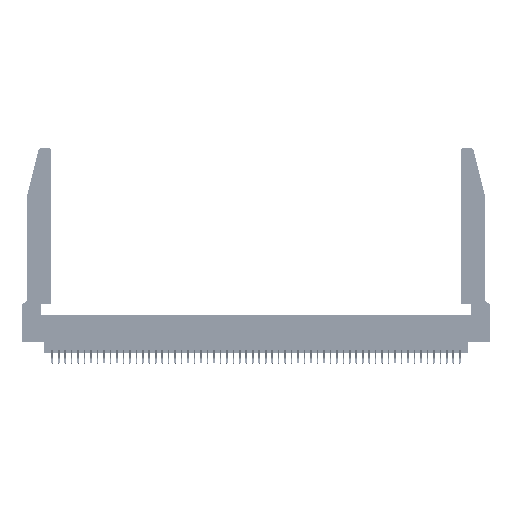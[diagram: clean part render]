
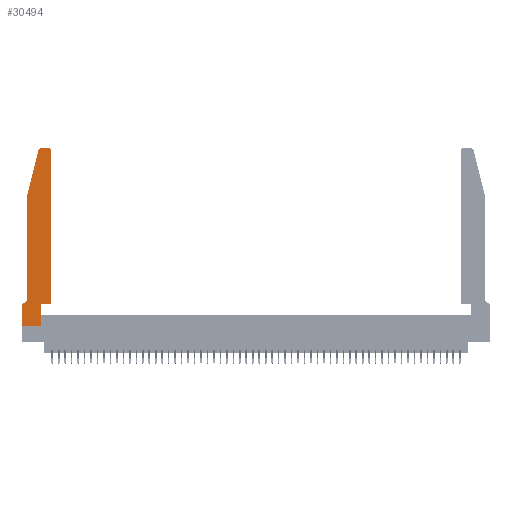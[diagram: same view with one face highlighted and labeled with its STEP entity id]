
A CAD part, top view. The second image highlights one B-rep face of the part: STEP entity #30494.
In plain terms, the highlighted planar face has unit normal (0, 0, 1).
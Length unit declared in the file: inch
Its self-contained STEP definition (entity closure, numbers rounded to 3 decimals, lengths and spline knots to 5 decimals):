
#531 = EDGE_CURVE ( 'NONE', #18446, #40915, #42597, .T. ) ;
#561 = ORIENTED_EDGE ( 'NONE', *, *, #23135, .T. ) ;
#687 = ORIENTED_EDGE ( 'NONE', *, *, #11111, .T. ) ;
#2513 = ORIENTED_EDGE ( 'NONE', *, *, #46568, .T. ) ;
#2864 = LINE ( 'NONE', #10462, #12907 ) ;
#4147 = CIRCLE ( 'NONE', #18333, 0.07 ) ;
#4244 = VECTOR ( 'NONE', #49688, 39.37008 ) ;
#4276 = DIRECTION ( 'NONE',  ( 0., 1., 0. ) ) ;
#4467 = CARTESIAN_POINT ( 'NONE',  ( 0.4205, 2.72, 0.37 ) ) ;
#5077 = CARTESIAN_POINT ( 'NONE',  ( 0.0755, 0.35, 0.37 ) ) ;
#5909 = VECTOR ( 'NONE', #18284, 39.37008 ) ;
#6375 = ORIENTED_EDGE ( 'NONE', *, *, #531, .T. ) ;
#6644 = AXIS2_PLACEMENT_3D ( 'NONE', #11214, #19170, #7177 ) ;
#6921 = DIRECTION ( 'NONE',  ( 1., 0., 0. ) ) ;
#7177 = DIRECTION ( 'NONE',  ( 1., 0., 0. ) ) ;
#7251 = ORIENTED_EDGE ( 'NONE', *, *, #20169, .T. ) ;
#7754 = CARTESIAN_POINT ( 'NONE',  ( 0.4505, 0.35, 0.37 ) ) ;
#7793 = EDGE_CURVE ( 'NONE', #28398, #52288, #38190, .T. ) ;
#8752 = CARTESIAN_POINT ( 'NONE',  ( 0., 0.35, 0.37 ) ) ;
#10229 = VERTEX_POINT ( 'NONE', #35747 ) ;
#10462 = CARTESIAN_POINT ( 'NONE',  ( 0., 0., 0.37 ) ) ;
#11111 = EDGE_CURVE ( 'NONE', #30848, #43019, #2864, .T. ) ;
#11214 = CARTESIAN_POINT ( 'NONE',  ( 0., 0.35, 0.37 ) ) ;
#12907 = VECTOR ( 'NONE', #23030, 39.37008 ) ;
#13020 = DIRECTION ( 'NONE',  ( -1., 0., 0. ) ) ;
#13340 = ORIENTED_EDGE ( 'NONE', *, *, #48735, .T. ) ;
#15078 = VECTOR ( 'NONE', #4276, 39.37008 ) ;
#15363 = CARTESIAN_POINT ( 'NONE',  ( 0.0755, 2., 0.37 ) ) ;
#16122 = CARTESIAN_POINT ( 'NONE',  ( 0.0755, 2., 0.37 ) ) ;
#16794 = EDGE_CURVE ( 'NONE', #52288, #40563, #49364, .T. ) ;
#16903 = EDGE_CURVE ( 'NONE', #34697, #10229, #19026, .T. ) ;
#18088 = LINE ( 'NONE', #5077, #35847 ) ;
#18284 = DIRECTION ( 'NONE',  ( 0., 1., 0. ) ) ;
#18333 = AXIS2_PLACEMENT_3D ( 'NONE', #35496, #46964, #51045 ) ;
#18446 = VERTEX_POINT ( 'NONE', #7754 ) ;
#18973 = CARTESIAN_POINT ( 'NONE',  ( 0.4505, 0.35, 0.37 ) ) ;
#19026 = LINE ( 'NONE', #41815, #30391 ) ;
#19170 = DIRECTION ( 'NONE',  ( 0., 0., 1. ) ) ;
#20121 = ORIENTED_EDGE ( 'NONE', *, *, #16794, .T. ) ;
#20169 = EDGE_CURVE ( 'NONE', #41918, #18446, #46542, .T. ) ;
#20224 = DIRECTION ( 'NONE',  ( -0.239, -0.971, 0. ) ) ;
#22528 = CARTESIAN_POINT ( 'NONE',  ( 0.0055, 0.35, 0.37 ) ) ;
#22739 = CARTESIAN_POINT ( 'NONE',  ( 0.2865, 0.35, 0.37 ) ) ;
#22975 = VECTOR ( 'NONE', #20224, 39.37008 ) ;
#23030 = DIRECTION ( 'NONE',  ( 1., 0., 0. ) ) ;
#23135 = EDGE_CURVE ( 'NONE', #46210, #30848, #42848, .T. ) ;
#23597 = PLANE ( 'NONE',  #6644 ) ;
#24251 = EDGE_CURVE ( 'NONE', #40563, #48288, #4147, .T. ) ;
#24945 = DIRECTION ( 'NONE',  ( 0., 0., 1. ) ) ;
#25653 = VECTOR ( 'NONE', #6921, 39.37008 ) ;
#26366 = AXIS2_PLACEMENT_3D ( 'NONE', #4467, #24945, #44942 ) ;
#26538 = DIRECTION ( 'NONE',  ( 0., -1., 0. ) ) ;
#27041 = CARTESIAN_POINT ( 'NONE',  ( 0.4505, 0.35, 0.37 ) ) ;
#27242 = ORIENTED_EDGE ( 'NONE', *, *, #51098, .T. ) ;
#28184 = EDGE_LOOP ( 'NONE', ( #50479, #2513, #41873, #20121, #33428, #27242, #561, #687, #13340, #7251, #6375, #51823 ) ) ;
#28398 = VERTEX_POINT ( 'NONE', #32281 ) ;
#28802 = CARTESIAN_POINT ( 'NONE',  ( 0., 0., 0.37 ) ) ;
#30045 = CARTESIAN_POINT ( 'NONE',  ( 0.0755, 0.42, 0.37 ) ) ;
#30391 = VECTOR ( 'NONE', #46049, 39.37008 ) ;
#30486 = CARTESIAN_POINT ( 'NONE',  ( 0.284, 2.72, 0.37 ) ) ;
#30494 = ADVANCED_FACE ( 'NONE', ( #31846 ), #23597, .T. ) ;
#30787 = CIRCLE ( 'NONE', #46043, 0.03 ) ;
#30823 = DIRECTION ( 'NONE',  ( 1., 0., 0. ) ) ;
#30848 = VERTEX_POINT ( 'NONE', #37529 ) ;
#31846 = FACE_OUTER_BOUND ( 'NONE', #28184, .T. ) ;
#32281 = CARTESIAN_POINT ( 'NONE',  ( 0.25487, 2.72718, 0.37 ) ) ;
#33246 = CARTESIAN_POINT ( 'NONE',  ( 0.2865, 0.35, 0.37 ) ) ;
#33428 = ORIENTED_EDGE ( 'NONE', *, *, #24251, .T. ) ;
#34697 = VERTEX_POINT ( 'NONE', #34959 ) ;
#34959 = CARTESIAN_POINT ( 'NONE',  ( 0.4205, 2.75, 0.37 ) ) ;
#35496 = CARTESIAN_POINT ( 'NONE',  ( 0.0055, 0.42, 0.37 ) ) ;
#35747 = CARTESIAN_POINT ( 'NONE',  ( 0.284, 2.75, 0.37 ) ) ;
#35847 = VECTOR ( 'NONE', #13020, 39.37008 ) ;
#37529 = CARTESIAN_POINT ( 'NONE',  ( 0., 0., 0.37 ) ) ;
#38190 = LINE ( 'NONE', #16122, #22975 ) ;
#40563 = VERTEX_POINT ( 'NONE', #30045 ) ;
#40915 = VERTEX_POINT ( 'NONE', #44369 ) ;
#41815 = CARTESIAN_POINT ( 'NONE',  ( 0.2605, 2.75, 0.37 ) ) ;
#41873 = ORIENTED_EDGE ( 'NONE', *, *, #7793, .T. ) ;
#41918 = VERTEX_POINT ( 'NONE', #22739 ) ;
#42597 = LINE ( 'NONE', #18973, #5909 ) ;
#42605 = CARTESIAN_POINT ( 'NONE',  ( 0.2865, 0., 0.37 ) ) ;
#42848 = LINE ( 'NONE', #28802, #4244 ) ;
#42857 = DIRECTION ( 'NONE',  ( 0., 0., 1. ) ) ;
#43019 = VERTEX_POINT ( 'NONE', #42605 ) ;
#44227 = LINE ( 'NONE', #33246, #15078 ) ;
#44369 = CARTESIAN_POINT ( 'NONE',  ( 0.4505, 2.72, 0.37 ) ) ;
#44942 = DIRECTION ( 'NONE',  ( 1., 0., 0. ) ) ;
#45626 = EDGE_CURVE ( 'NONE', #40915, #34697, #50483, .T. ) ;
#46043 = AXIS2_PLACEMENT_3D ( 'NONE', #30486, #42857, #30823 ) ;
#46049 = DIRECTION ( 'NONE',  ( -1., 0., 0. ) ) ;
#46210 = VERTEX_POINT ( 'NONE', #8752 ) ;
#46212 = VECTOR ( 'NONE', #26538, 39.37008 ) ;
#46542 = LINE ( 'NONE', #27041, #25653 ) ;
#46568 = EDGE_CURVE ( 'NONE', #10229, #28398, #30787, .T. ) ;
#46964 = DIRECTION ( 'NONE',  ( 0., 0., -1. ) ) ;
#47494 = CARTESIAN_POINT ( 'NONE',  ( 0.0755, 2., 0.37 ) ) ;
#48288 = VERTEX_POINT ( 'NONE', #22528 ) ;
#48735 = EDGE_CURVE ( 'NONE', #43019, #41918, #44227, .T. ) ;
#49364 = LINE ( 'NONE', #47494, #46212 ) ;
#49688 = DIRECTION ( 'NONE',  ( 0., -1., 0. ) ) ;
#50479 = ORIENTED_EDGE ( 'NONE', *, *, #16903, .T. ) ;
#50483 = CIRCLE ( 'NONE', #26366, 0.03 ) ;
#51045 = DIRECTION ( 'NONE',  ( -1., 0., 0. ) ) ;
#51098 = EDGE_CURVE ( 'NONE', #48288, #46210, #18088, .T. ) ;
#51823 = ORIENTED_EDGE ( 'NONE', *, *, #45626, .T. ) ;
#52288 = VERTEX_POINT ( 'NONE', #15363 ) ;
